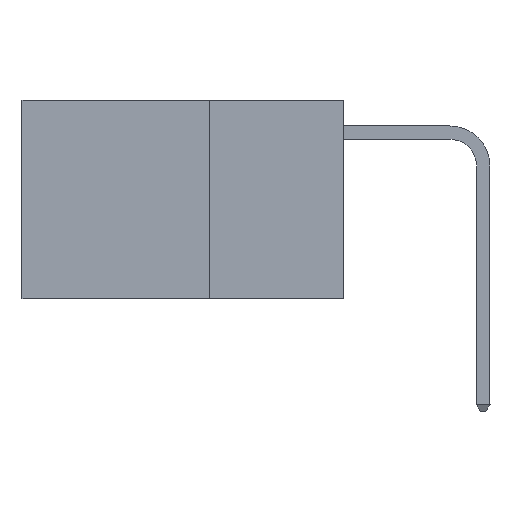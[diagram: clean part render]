
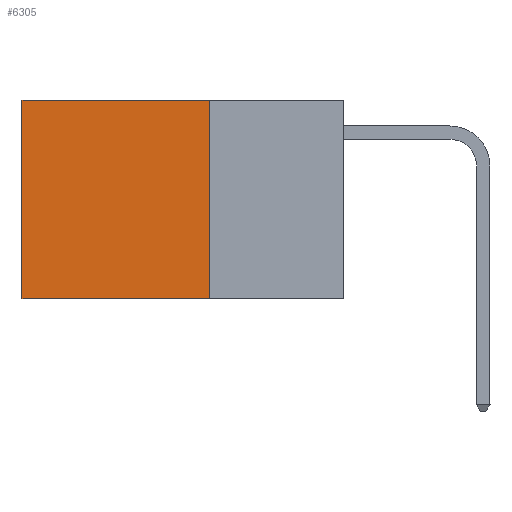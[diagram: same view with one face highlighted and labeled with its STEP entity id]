
A CAD part, left-side view. The second image highlights one B-rep face of the part: STEP entity #6305.
In plain terms, the highlighted planar face has unit normal (-1, 0, 0).
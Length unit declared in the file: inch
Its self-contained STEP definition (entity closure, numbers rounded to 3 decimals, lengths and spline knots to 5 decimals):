
#190 = VECTOR ( 'NONE', #7053, 39.37008 ) ;
#227 = AXIS2_PLACEMENT_3D ( 'NONE', #9881, #2619, #12869 ) ;
#616 = VERTEX_POINT ( 'NONE', #1446 ) ;
#740 = PLANE ( 'NONE',  #227 ) ;
#900 = EDGE_CURVE ( 'NONE', #4203, #1815, #12844, .T. ) ;
#1446 = CARTESIAN_POINT ( 'NONE',  ( 0.2625, 0.25, 0. ) ) ;
#1815 = VERTEX_POINT ( 'NONE', #6217 ) ;
#1818 = CARTESIAN_POINT ( 'NONE',  ( 0.2625, 0.25, 0. ) ) ;
#2619 = DIRECTION ( 'NONE',  ( 1., 0., 0. ) ) ;
#3095 = EDGE_CURVE ( 'NONE', #616, #4203, #6104, .T. ) ;
#3679 = CARTESIAN_POINT ( 'NONE',  ( 0.2625, 0.6, 0. ) ) ;
#3906 = LINE ( 'NONE', #9034, #12709 ) ;
#4203 = VERTEX_POINT ( 'NONE', #5307 ) ;
#4786 = VECTOR ( 'NONE', #11242, 39.37008 ) ;
#4896 = ORIENTED_EDGE ( 'NONE', *, *, #10244, .F. ) ;
#5307 = CARTESIAN_POINT ( 'NONE',  ( 0.2625, 0.6, 0. ) ) ;
#5605 = CARTESIAN_POINT ( 'NONE',  ( 0.2625, 0.25, -0.37 ) ) ;
#6063 = DIRECTION ( 'NONE',  ( 0., 0., -1. ) ) ;
#6104 = LINE ( 'NONE', #1818, #190 ) ;
#6217 = CARTESIAN_POINT ( 'NONE',  ( 0.2625, 0.6, -0.37 ) ) ;
#6305 = ADVANCED_FACE ( 'NONE', ( #7654 ), #740, .F. ) ;
#7053 = DIRECTION ( 'NONE',  ( 0., 1., 0. ) ) ;
#7654 = FACE_OUTER_BOUND ( 'NONE', #11778, .T. ) ;
#8209 = CARTESIAN_POINT ( 'NONE',  ( 0.2625, 0.25, -0.37 ) ) ;
#8385 = ORIENTED_EDGE ( 'NONE', *, *, #3095, .T. ) ;
#8546 = ORIENTED_EDGE ( 'NONE', *, *, #900, .T. ) ;
#8875 = VECTOR ( 'NONE', #6063, 39.37008 ) ;
#9034 = CARTESIAN_POINT ( 'NONE',  ( 0.2625, 0.25, 0. ) ) ;
#9167 = DIRECTION ( 'NONE',  ( 0., 0., -1. ) ) ;
#9470 = VERTEX_POINT ( 'NONE', #5605 ) ;
#9881 = CARTESIAN_POINT ( 'NONE',  ( 0.2625, 0.25, 0. ) ) ;
#10112 = EDGE_CURVE ( 'NONE', #616, #9470, #3906, .T. ) ;
#10244 = EDGE_CURVE ( 'NONE', #9470, #1815, #11512, .T. ) ;
#10375 = ORIENTED_EDGE ( 'NONE', *, *, #10112, .F. ) ;
#11242 = DIRECTION ( 'NONE',  ( 0., 1., 0. ) ) ;
#11512 = LINE ( 'NONE', #8209, #4786 ) ;
#11778 = EDGE_LOOP ( 'NONE', ( #8546, #4896, #10375, #8385 ) ) ;
#12709 = VECTOR ( 'NONE', #9167, 39.37008 ) ;
#12844 = LINE ( 'NONE', #3679, #8875 ) ;
#12869 = DIRECTION ( 'NONE',  ( 0., 0., -1. ) ) ;
